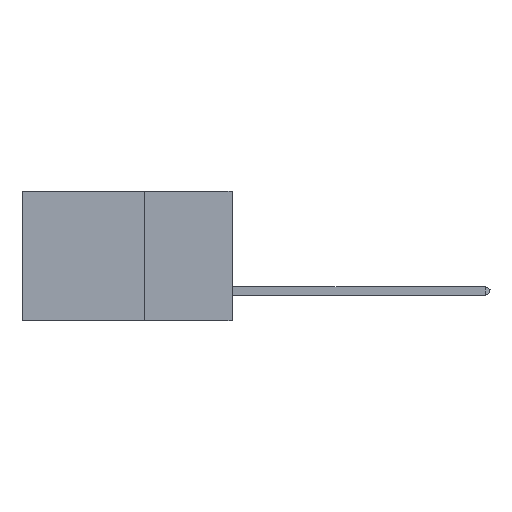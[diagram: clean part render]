
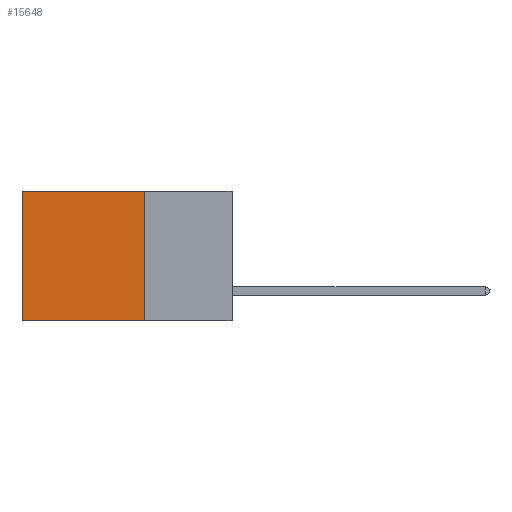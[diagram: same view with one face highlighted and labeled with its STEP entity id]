
A CAD part, left-side view. The second image highlights one B-rep face of the part: STEP entity #15648.
In plain terms, the highlighted planar face has unit normal (-1, 0, 0).
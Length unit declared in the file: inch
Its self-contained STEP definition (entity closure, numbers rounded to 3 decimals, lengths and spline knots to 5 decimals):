
#477 = VERTEX_POINT ( 'NONE', #18238 ) ;
#620 = CARTESIAN_POINT ( 'NONE',  ( 0.2875, 0.25, 0. ) ) ;
#715 = CARTESIAN_POINT ( 'NONE',  ( 0.2875, 0.25, 0. ) ) ;
#815 = VERTEX_POINT ( 'NONE', #3876 ) ;
#1026 = VECTOR ( 'NONE', #17114, 39.37008 ) ;
#1625 = ORIENTED_EDGE ( 'NONE', *, *, #6924, .T. ) ;
#2099 = CARTESIAN_POINT ( 'NONE',  ( 0.2875, 0.6, 0. ) ) ;
#2509 = DIRECTION ( 'NONE',  ( 0., 1., 0. ) ) ;
#3876 = CARTESIAN_POINT ( 'NONE',  ( 0.2875, 0.6, -0.37 ) ) ;
#5489 = EDGE_LOOP ( 'NONE', ( #1625, #14511, #11899, #6692 ) ) ;
#5535 = LINE ( 'NONE', #15369, #8561 ) ;
#5591 = DIRECTION ( 'NONE',  ( 0., 0., -1. ) ) ;
#6692 = ORIENTED_EDGE ( 'NONE', *, *, #16376, .T. ) ;
#6924 = EDGE_CURVE ( 'NONE', #477, #815, #21488, .T. ) ;
#7184 = EDGE_CURVE ( 'NONE', #10703, #20521, #5535, .T. ) ;
#7991 = DIRECTION ( 'NONE',  ( 0., 0., -1. ) ) ;
#8561 = VECTOR ( 'NONE', #7991, 39.37008 ) ;
#9975 = VECTOR ( 'NONE', #12841, 39.37008 ) ;
#10151 = CARTESIAN_POINT ( 'NONE',  ( 0.2875, 0.25, -0.37 ) ) ;
#10703 = VERTEX_POINT ( 'NONE', #715 ) ;
#11208 = DIRECTION ( 'NONE',  ( 1., 0., 0. ) ) ;
#11899 = ORIENTED_EDGE ( 'NONE', *, *, #7184, .F. ) ;
#12841 = DIRECTION ( 'NONE',  ( 0., 0., -1. ) ) ;
#12973 = PLANE ( 'NONE',  #20688 ) ;
#13010 = CARTESIAN_POINT ( 'NONE',  ( 0.2875, 0.25, 0. ) ) ;
#13964 = EDGE_CURVE ( 'NONE', #20521, #815, #19687, .T. ) ;
#14511 = ORIENTED_EDGE ( 'NONE', *, *, #13964, .F. ) ;
#15369 = CARTESIAN_POINT ( 'NONE',  ( 0.2875, 0.25, 0. ) ) ;
#15648 = ADVANCED_FACE ( 'NONE', ( #18787 ), #12973, .F. ) ;
#16376 = EDGE_CURVE ( 'NONE', #10703, #477, #17933, .T. ) ;
#17114 = DIRECTION ( 'NONE',  ( 0., 1., 0. ) ) ;
#17933 = LINE ( 'NONE', #13010, #20682 ) ;
#18238 = CARTESIAN_POINT ( 'NONE',  ( 0.2875, 0.6, 0. ) ) ;
#18594 = CARTESIAN_POINT ( 'NONE',  ( 0.2875, 0.25, -0.37 ) ) ;
#18787 = FACE_OUTER_BOUND ( 'NONE', #5489, .T. ) ;
#19687 = LINE ( 'NONE', #10151, #1026 ) ;
#20521 = VERTEX_POINT ( 'NONE', #18594 ) ;
#20682 = VECTOR ( 'NONE', #2509, 39.37008 ) ;
#20688 = AXIS2_PLACEMENT_3D ( 'NONE', #620, #11208, #5591 ) ;
#21488 = LINE ( 'NONE', #2099, #9975 ) ;
